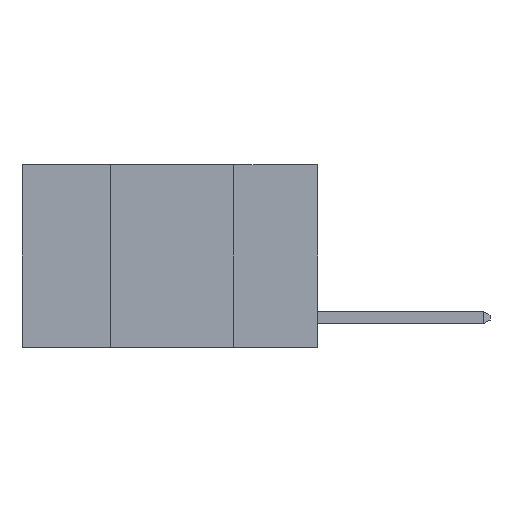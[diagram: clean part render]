
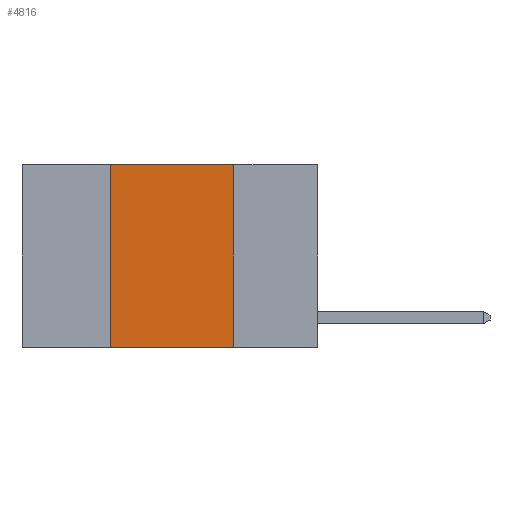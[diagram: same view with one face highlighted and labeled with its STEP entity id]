
A CAD part, left-side view. The second image highlights one B-rep face of the part: STEP entity #4816.
In plain terms, the highlighted planar face has unit normal (-1, 0, 0).
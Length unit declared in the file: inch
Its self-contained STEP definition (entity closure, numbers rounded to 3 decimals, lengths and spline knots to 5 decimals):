
#105 = AXIS2_PLACEMENT_3D ( 'NONE', #2955, #5578, #1674 ) ;
#192 = CARTESIAN_POINT ( 'NONE',  ( 0., 0.17, -0.37 ) ) ;
#231 = EDGE_CURVE ( 'NONE', #1654, #3511, #3371, .T. ) ;
#655 = LINE ( 'NONE', #3491, #4102 ) ;
#1119 = EDGE_CURVE ( 'NONE', #3511, #2728, #4378, .T. ) ;
#1478 = DIRECTION ( 'NONE',  ( 0., -1., 0. ) ) ;
#1611 = ORIENTED_EDGE ( 'NONE', *, *, #3439, .T. ) ;
#1654 = VERTEX_POINT ( 'NONE', #2977 ) ;
#1665 = VECTOR ( 'NONE', #7652, 39.37008 ) ;
#1674 = DIRECTION ( 'NONE',  ( 0., 0., -1. ) ) ;
#1863 = LINE ( 'NONE', #5517, #1665 ) ;
#2489 = VECTOR ( 'NONE', #1478, 39.37008 ) ;
#2728 = VERTEX_POINT ( 'NONE', #4430 ) ;
#2955 = CARTESIAN_POINT ( 'NONE',  ( 0., 0.6, 0. ) ) ;
#2977 = CARTESIAN_POINT ( 'NONE',  ( 0., 0.42, -0.37 ) ) ;
#3025 = ORIENTED_EDGE ( 'NONE', *, *, #231, .F. ) ;
#3371 = LINE ( 'NONE', #5475, #8191 ) ;
#3439 = EDGE_CURVE ( 'NONE', #1654, #7428, #1863, .T. ) ;
#3491 = CARTESIAN_POINT ( 'NONE',  ( 0., 0.17, 0. ) ) ;
#3511 = VERTEX_POINT ( 'NONE', #5002 ) ;
#4102 = VECTOR ( 'NONE', #4155, 39.37008 ) ;
#4126 = ORIENTED_EDGE ( 'NONE', *, *, #6767, .F. ) ;
#4155 = DIRECTION ( 'NONE',  ( 0., 0., -1. ) ) ;
#4378 = LINE ( 'NONE', #5559, #2489 ) ;
#4430 = CARTESIAN_POINT ( 'NONE',  ( 0., 0.17, 0. ) ) ;
#4816 = ADVANCED_FACE ( 'NONE', ( #4846 ), #4882, .F. ) ;
#4846 = FACE_OUTER_BOUND ( 'NONE', #5399, .T. ) ;
#4882 = PLANE ( 'NONE',  #105 ) ;
#5002 = CARTESIAN_POINT ( 'NONE',  ( 0., 0.42, 0. ) ) ;
#5399 = EDGE_LOOP ( 'NONE', ( #4126, #6488, #3025, #1611 ) ) ;
#5475 = CARTESIAN_POINT ( 'NONE',  ( 0., 0.42, 0. ) ) ;
#5517 = CARTESIAN_POINT ( 'NONE',  ( 0., 0.6, -0.37 ) ) ;
#5559 = CARTESIAN_POINT ( 'NONE',  ( 0., 0.6, 0. ) ) ;
#5578 = DIRECTION ( 'NONE',  ( 1., 0., 0. ) ) ;
#5710 = DIRECTION ( 'NONE',  ( 0., 0., 1. ) ) ;
#6488 = ORIENTED_EDGE ( 'NONE', *, *, #1119, .F. ) ;
#6767 = EDGE_CURVE ( 'NONE', #2728, #7428, #655, .T. ) ;
#7428 = VERTEX_POINT ( 'NONE', #192 ) ;
#7652 = DIRECTION ( 'NONE',  ( 0., -1., 0. ) ) ;
#8191 = VECTOR ( 'NONE', #5710, 39.37008 ) ;
